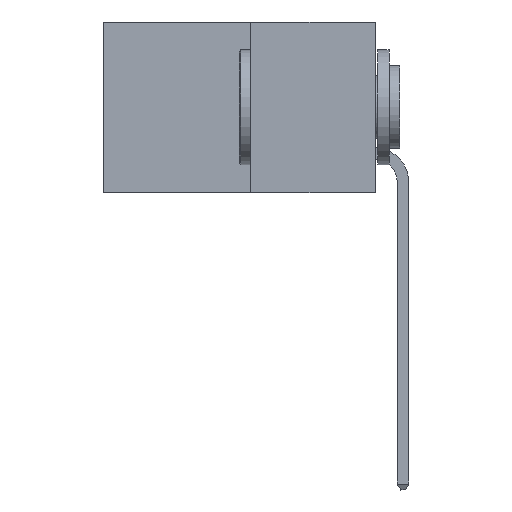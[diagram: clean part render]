
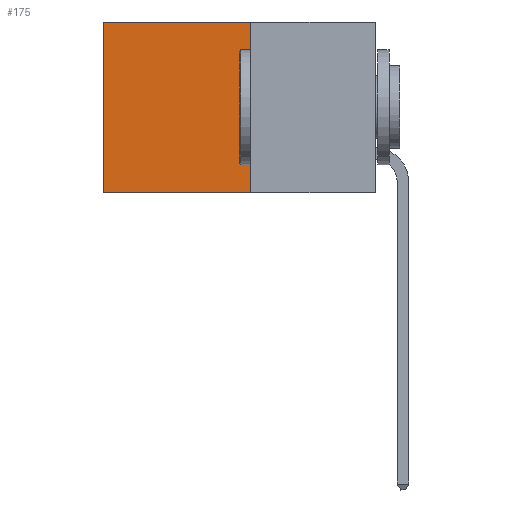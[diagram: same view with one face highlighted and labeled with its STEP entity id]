
A CAD part, left-side view. The second image highlights one B-rep face of the part: STEP entity #175.
In plain terms, the highlighted planar face has unit normal (-1, 0, 0).
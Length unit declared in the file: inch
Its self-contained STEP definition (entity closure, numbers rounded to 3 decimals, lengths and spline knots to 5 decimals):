
#95 = CARTESIAN_POINT ( 'NONE',  ( 0.277, 0.27, 0. ) ) ;
#175 = ADVANCED_FACE ( 'NONE', ( #3452 ), #9435, .F. ) ;
#335 = VERTEX_POINT ( 'NONE', #5890 ) ;
#1254 = DIRECTION ( 'NONE',  ( 0., 1., 0. ) ) ;
#2018 = ORIENTED_EDGE ( 'NONE', *, *, #6134, .T. ) ;
#2324 = ORIENTED_EDGE ( 'NONE', *, *, #11902, .F. ) ;
#2636 = ORIENTED_EDGE ( 'NONE', *, *, #3496, .F. ) ;
#3452 = FACE_OUTER_BOUND ( 'NONE', #12223, .T. ) ;
#3496 = EDGE_CURVE ( 'NONE', #11797, #335, #4817, .T. ) ;
#3851 = DIRECTION ( 'NONE',  ( 0., 0., -1. ) ) ;
#4032 = DIRECTION ( 'NONE',  ( 0., 0., -1. ) ) ;
#4251 = CARTESIAN_POINT ( 'NONE',  ( 0.277, 0.27, -0.37 ) ) ;
#4276 = VECTOR ( 'NONE', #3851, 39.37008 ) ;
#4817 = LINE ( 'NONE', #5972, #7254 ) ;
#5782 = EDGE_CURVE ( 'NONE', #11797, #7610, #12910, .T. ) ;
#5890 = CARTESIAN_POINT ( 'NONE',  ( 0.277, 0.27, -0.37 ) ) ;
#5972 = CARTESIAN_POINT ( 'NONE',  ( 0.277, 0.27, -0.37 ) ) ;
#6134 = EDGE_CURVE ( 'NONE', #7610, #8507, #7389, .T. ) ;
#6679 = LINE ( 'NONE', #4251, #11649 ) ;
#7254 = VECTOR ( 'NONE', #4032, 39.37008 ) ;
#7389 = LINE ( 'NONE', #10022, #4276 ) ;
#7402 = DIRECTION ( 'NONE',  ( 0., 1., 0. ) ) ;
#7610 = VERTEX_POINT ( 'NONE', #8406 ) ;
#7982 = DIRECTION ( 'NONE',  ( 0., 0., -1. ) ) ;
#8132 = ORIENTED_EDGE ( 'NONE', *, *, #5782, .T. ) ;
#8406 = CARTESIAN_POINT ( 'NONE',  ( 0.277, 0.59, 0. ) ) ;
#8507 = VERTEX_POINT ( 'NONE', #12047 ) ;
#8623 = DIRECTION ( 'NONE',  ( 1., 0., 0. ) ) ;
#9328 = CARTESIAN_POINT ( 'NONE',  ( 0.277, 0.27, -0.37 ) ) ;
#9435 = PLANE ( 'NONE',  #11723 ) ;
#10022 = CARTESIAN_POINT ( 'NONE',  ( 0.277, 0.59, -0.37 ) ) ;
#11649 = VECTOR ( 'NONE', #7402, 39.37008 ) ;
#11723 = AXIS2_PLACEMENT_3D ( 'NONE', #9328, #8623, #7982 ) ;
#11797 = VERTEX_POINT ( 'NONE', #12128 ) ;
#11902 = EDGE_CURVE ( 'NONE', #335, #8507, #6679, .T. ) ;
#12047 = CARTESIAN_POINT ( 'NONE',  ( 0.277, 0.59, -0.37 ) ) ;
#12128 = CARTESIAN_POINT ( 'NONE',  ( 0.277, 0.27, 0. ) ) ;
#12223 = EDGE_LOOP ( 'NONE', ( #2018, #2324, #2636, #8132 ) ) ;
#12326 = VECTOR ( 'NONE', #1254, 39.37008 ) ;
#12910 = LINE ( 'NONE', #95, #12326 ) ;
